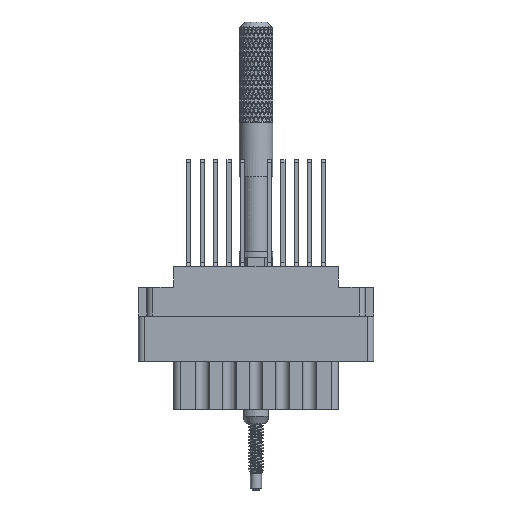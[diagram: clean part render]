
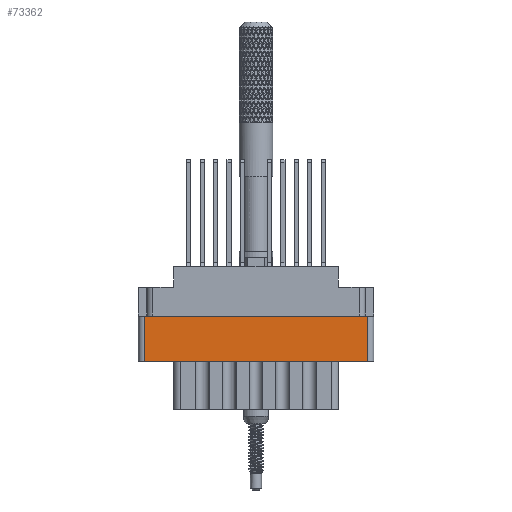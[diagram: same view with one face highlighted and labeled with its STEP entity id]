
A CAD part, front view. The second image highlights one B-rep face of the part: STEP entity #73362.
In plain terms, the highlighted planar face has unit normal (0, -1, 0).
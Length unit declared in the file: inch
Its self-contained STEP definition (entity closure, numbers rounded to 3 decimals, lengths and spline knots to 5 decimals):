
#985 = AXIS2_PLACEMENT_3D ( 'NONE', #159572, #117075, #30263 ) ;
#4690 = VECTOR ( 'NONE', #127038, 39.37008 ) ;
#6256 = ORIENTED_EDGE ( 'NONE', *, *, #135189, .T. ) ;
#8755 = VECTOR ( 'NONE', #84855, 39.37008 ) ;
#9870 = EDGE_CURVE ( 'NONE', #25440, #49976, #38133, .T. ) ;
#22088 = DIRECTION ( 'NONE',  ( 0., 0., -1. ) ) ;
#25001 = LINE ( 'NONE', #42662, #4690 ) ;
#25440 = VERTEX_POINT ( 'NONE', #185154 ) ;
#30263 = DIRECTION ( 'NONE',  ( 0., 0., -1. ) ) ;
#38133 = LINE ( 'NONE', #84228, #8755 ) ;
#42662 = CARTESIAN_POINT ( 'NONE',  ( 0., -0.343, -0.529 ) ) ;
#49976 = VERTEX_POINT ( 'NONE', #173326 ) ;
#61236 = CARTESIAN_POINT ( 'NONE',  ( 0., -0.343, -0.277 ) ) ;
#63491 = LINE ( 'NONE', #61236, #97492 ) ;
#73362 = ADVANCED_FACE ( 'NONE', ( #115949 ), #118300, .T. ) ;
#74685 = VECTOR ( 'NONE', #22088, 39.37008 ) ;
#77014 = DIRECTION ( 'NONE',  ( 1., 0., 0. ) ) ;
#77843 = CARTESIAN_POINT ( 'NONE',  ( -0.624, -0.343, -0.277 ) ) ;
#79321 = EDGE_CURVE ( 'NONE', #141631, #49976, #63491, .T. ) ;
#80927 = CARTESIAN_POINT ( 'NONE',  ( -0.624, -0.343, -0.798 ) ) ;
#84197 = CARTESIAN_POINT ( 'NONE',  ( -0.624, -0.343, -0.529 ) ) ;
#84228 = CARTESIAN_POINT ( 'NONE',  ( 0.624, -0.343, -0.798 ) ) ;
#84855 = DIRECTION ( 'NONE',  ( 0., 0., 1. ) ) ;
#91913 = ORIENTED_EDGE ( 'NONE', *, *, #79321, .F. ) ;
#97492 = VECTOR ( 'NONE', #77014, 39.37008 ) ;
#115949 = FACE_OUTER_BOUND ( 'NONE', #185785, .T. ) ;
#116226 = ORIENTED_EDGE ( 'NONE', *, *, #9870, .T. ) ;
#117075 = DIRECTION ( 'NONE',  ( 0., -1., 0. ) ) ;
#118300 = PLANE ( 'NONE',  #985 ) ;
#126451 = ORIENTED_EDGE ( 'NONE', *, *, #178067, .F. ) ;
#127038 = DIRECTION ( 'NONE',  ( -1., 0., 0. ) ) ;
#135189 = EDGE_CURVE ( 'NONE', #141631, #174595, #181216, .T. ) ;
#141631 = VERTEX_POINT ( 'NONE', #77843 ) ;
#159572 = CARTESIAN_POINT ( 'NONE',  ( -0.656, -0.343, -0.798 ) ) ;
#173326 = CARTESIAN_POINT ( 'NONE',  ( 0.624, -0.343, -0.277 ) ) ;
#174595 = VERTEX_POINT ( 'NONE', #84197 ) ;
#178067 = EDGE_CURVE ( 'NONE', #25440, #174595, #25001, .T. ) ;
#181216 = LINE ( 'NONE', #80927, #74685 ) ;
#185154 = CARTESIAN_POINT ( 'NONE',  ( 0.624, -0.343, -0.529 ) ) ;
#185785 = EDGE_LOOP ( 'NONE', ( #91913, #6256, #126451, #116226 ) ) ;
